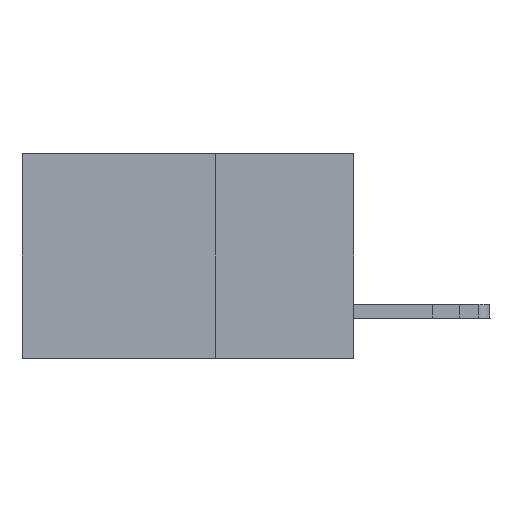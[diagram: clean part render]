
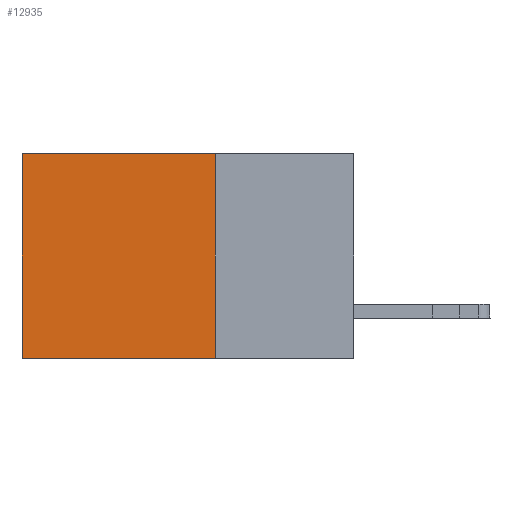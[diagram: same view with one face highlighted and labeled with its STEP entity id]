
A CAD part, left-side view. The second image highlights one B-rep face of the part: STEP entity #12935.
In plain terms, the highlighted planar face has unit normal (-1, 0, 0).
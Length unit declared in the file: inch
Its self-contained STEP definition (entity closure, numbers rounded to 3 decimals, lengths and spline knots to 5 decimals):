
#811 = DIRECTION ( 'NONE',  ( 0., 1., 0. ) ) ;
#2195 = AXIS2_PLACEMENT_3D ( 'NONE', #7090, #9345, #18151 ) ;
#2581 = DIRECTION ( 'NONE',  ( 0., 0., -1. ) ) ;
#2735 = ORIENTED_EDGE ( 'NONE', *, *, #4037, .F. ) ;
#2809 = CARTESIAN_POINT ( 'NONE',  ( 0.2875, 0.25, -0.37 ) ) ;
#3574 = CARTESIAN_POINT ( 'NONE',  ( 0.2875, 0.6, 0. ) ) ;
#3664 = EDGE_CURVE ( 'NONE', #4527, #22088, #8163, .T. ) ;
#4037 = EDGE_CURVE ( 'NONE', #15688, #8518, #7858, .T. ) ;
#4176 = DIRECTION ( 'NONE',  ( 0., 1., 0. ) ) ;
#4527 = VERTEX_POINT ( 'NONE', #8813 ) ;
#6687 = EDGE_CURVE ( 'NONE', #22088, #8518, #16770, .T. ) ;
#7090 = CARTESIAN_POINT ( 'NONE',  ( 0.2875, 0.25, 0. ) ) ;
#7521 = CARTESIAN_POINT ( 'NONE',  ( 0.2875, 0.6, -0.37 ) ) ;
#7654 = FACE_OUTER_BOUND ( 'NONE', #13209, .T. ) ;
#7858 = LINE ( 'NONE', #11282, #9613 ) ;
#8163 = LINE ( 'NONE', #21201, #15461 ) ;
#8518 = VERTEX_POINT ( 'NONE', #7521 ) ;
#8813 = CARTESIAN_POINT ( 'NONE',  ( 0.2875, 0.25, 0. ) ) ;
#9345 = DIRECTION ( 'NONE',  ( 1., 0., 0. ) ) ;
#9613 = VECTOR ( 'NONE', #4176, 39.37008 ) ;
#9813 = VECTOR ( 'NONE', #2581, 39.37008 ) ;
#9977 = ORIENTED_EDGE ( 'NONE', *, *, #6687, .T. ) ;
#11282 = CARTESIAN_POINT ( 'NONE',  ( 0.2875, 0.25, -0.37 ) ) ;
#12508 = PLANE ( 'NONE',  #2195 ) ;
#12565 = ORIENTED_EDGE ( 'NONE', *, *, #15865, .F. ) ;
#12730 = ORIENTED_EDGE ( 'NONE', *, *, #3664, .T. ) ;
#12935 = ADVANCED_FACE ( 'NONE', ( #7654 ), #12508, .F. ) ;
#13014 = VECTOR ( 'NONE', #15202, 39.37008 ) ;
#13027 = CARTESIAN_POINT ( 'NONE',  ( 0.2875, 0.25, 0. ) ) ;
#13209 = EDGE_LOOP ( 'NONE', ( #9977, #2735, #12565, #12730 ) ) ;
#15028 = LINE ( 'NONE', #13027, #13014 ) ;
#15202 = DIRECTION ( 'NONE',  ( 0., 0., -1. ) ) ;
#15461 = VECTOR ( 'NONE', #811, 39.37008 ) ;
#15688 = VERTEX_POINT ( 'NONE', #2809 ) ;
#15865 = EDGE_CURVE ( 'NONE', #4527, #15688, #15028, .T. ) ;
#16770 = LINE ( 'NONE', #23427, #9813 ) ;
#18151 = DIRECTION ( 'NONE',  ( 0., 0., -1. ) ) ;
#21201 = CARTESIAN_POINT ( 'NONE',  ( 0.2875, 0.25, 0. ) ) ;
#22088 = VERTEX_POINT ( 'NONE', #3574 ) ;
#23427 = CARTESIAN_POINT ( 'NONE',  ( 0.2875, 0.6, 0. ) ) ;
